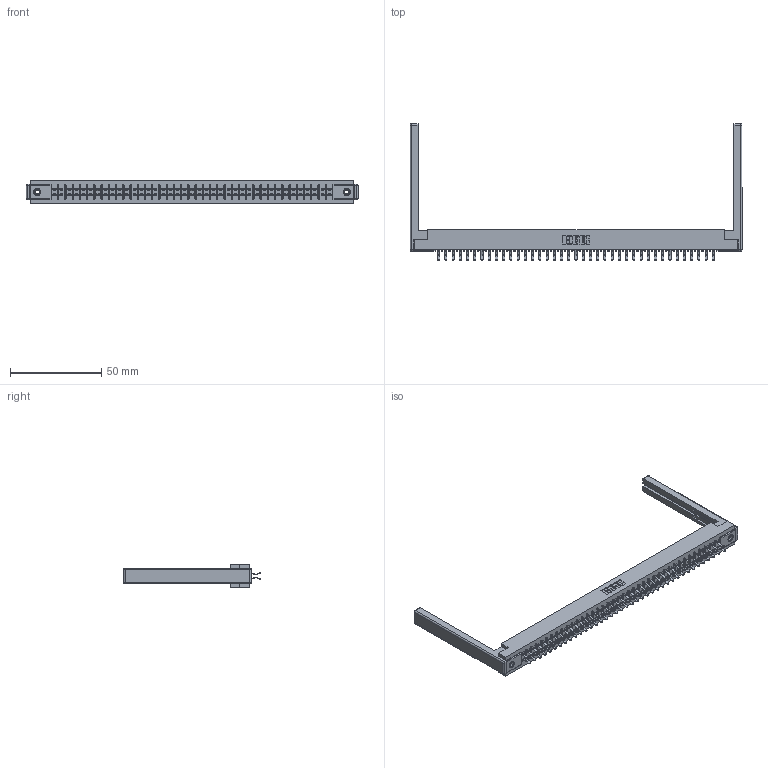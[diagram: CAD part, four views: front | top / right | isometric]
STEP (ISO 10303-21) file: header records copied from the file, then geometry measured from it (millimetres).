
FILE_DESCRIPTION (( 'STEP AP203' ), '1' );
FILE_NAME ('305-078-556-568.STEP', '2019-09-10T09:29:40', ( '' ), ( '' ), 'SwSTEP 2.0', 'SolidWorks 2016', '' );
FILE_SCHEMA (( 'CONFIG_CONTROL_DESIGN' ));
Length unit declared in the file: inch
Products named in the file (5): 345-250-001_345-250-001-102; 305 Part_.156 Dia; 305-078-556-568; 305-290-001_556; 307-220-068
Assembly tree (83 placements, depth 2):
  305-078-556-568
    305 Part_.156 Dia
    305-290-001_556  x78
    345-250-001_345-250-001-102  x2
    307-220-068  x2
Bounding box: 181.97 x 74.93 x 12.7 mm (x, y, z)
Volume: 22804 mm3; surface area: 28218 mm2
Topology: 83 solids, 83 shells, 4638 faces, 13303 edges, 8638 vertices
Faces by surface type: plane 2574, cylinder 1884, sphere 164, cone 12, torus 4
Entity records: 45573 total; most frequent: CARTESIAN_POINT 7516, ORIENTED_EDGE 7452, DIRECTION 7296, EDGE_CURVE 3726, VECTOR 2996, LINE 2996, VERTEX_POINT 2370, AXIS2_PLACEMENT_3D 2150
